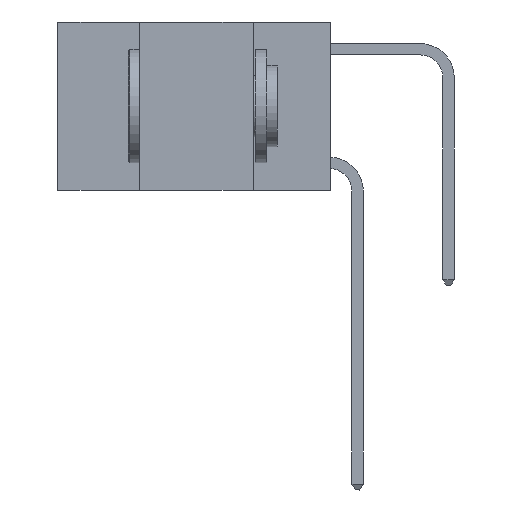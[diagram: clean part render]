
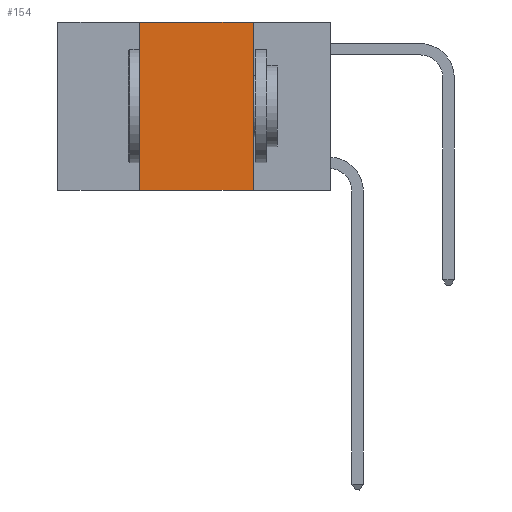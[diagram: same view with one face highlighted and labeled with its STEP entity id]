
A CAD part, left-side view. The second image highlights one B-rep face of the part: STEP entity #154.
In plain terms, the highlighted planar face has unit normal (-1, 0, 0).
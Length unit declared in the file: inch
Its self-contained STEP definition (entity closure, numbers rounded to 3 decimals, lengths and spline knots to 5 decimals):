
#154 = ADVANCED_FACE ( 'NONE', ( #8754 ), #3872, .F. ) ;
#316 = DIRECTION ( 'NONE',  ( 0., -1., 0. ) ) ;
#489 = LINE ( 'NONE', #976, #1999 ) ;
#568 = DIRECTION ( 'NONE',  ( 0., 0., -1. ) ) ;
#976 = CARTESIAN_POINT ( 'NONE',  ( 0., 0.42, 0. ) ) ;
#1014 = DIRECTION ( 'NONE',  ( 0., -1., 0. ) ) ;
#1999 = VECTOR ( 'NONE', #2169, 39.37008 ) ;
#2169 = DIRECTION ( 'NONE',  ( 0., 0., 1. ) ) ;
#2702 = VERTEX_POINT ( 'NONE', #7070 ) ;
#2782 = DIRECTION ( 'NONE',  ( 0., 0., -1. ) ) ;
#3021 = VERTEX_POINT ( 'NONE', #5726 ) ;
#3030 = EDGE_CURVE ( 'NONE', #2702, #3021, #5321, .T. ) ;
#3393 = VECTOR ( 'NONE', #1014, 39.37008 ) ;
#3872 = PLANE ( 'NONE',  #5200 ) ;
#4169 = ORIENTED_EDGE ( 'NONE', *, *, #7814, .T. ) ;
#4462 = VECTOR ( 'NONE', #2782, 39.37008 ) ;
#4655 = VECTOR ( 'NONE', #316, 39.37008 ) ;
#5200 = AXIS2_PLACEMENT_3D ( 'NONE', #6971, #9347, #568 ) ;
#5321 = LINE ( 'NONE', #10060, #4655 ) ;
#5398 = CARTESIAN_POINT ( 'NONE',  ( 0., 0.17, 0. ) ) ;
#5475 = EDGE_LOOP ( 'NONE', ( #6475, #6229, #9011, #4169 ) ) ;
#5726 = CARTESIAN_POINT ( 'NONE',  ( 0., 0.17, 0. ) ) ;
#5914 = VERTEX_POINT ( 'NONE', #9217 ) ;
#6229 = ORIENTED_EDGE ( 'NONE', *, *, #3030, .F. ) ;
#6475 = ORIENTED_EDGE ( 'NONE', *, *, #11972, .F. ) ;
#6971 = CARTESIAN_POINT ( 'NONE',  ( 0., 0.6, 0. ) ) ;
#7070 = CARTESIAN_POINT ( 'NONE',  ( 0., 0.42, 0. ) ) ;
#7090 = LINE ( 'NONE', #7500, #3393 ) ;
#7315 = LINE ( 'NONE', #5398, #4462 ) ;
#7500 = CARTESIAN_POINT ( 'NONE',  ( 0., 0.6, -0.37 ) ) ;
#7814 = EDGE_CURVE ( 'NONE', #5914, #13122, #7090, .T. ) ;
#8754 = FACE_OUTER_BOUND ( 'NONE', #5475, .T. ) ;
#9011 = ORIENTED_EDGE ( 'NONE', *, *, #9287, .F. ) ;
#9217 = CARTESIAN_POINT ( 'NONE',  ( 0., 0.42, -0.37 ) ) ;
#9287 = EDGE_CURVE ( 'NONE', #5914, #2702, #489, .T. ) ;
#9347 = DIRECTION ( 'NONE',  ( 1., 0., 0. ) ) ;
#10060 = CARTESIAN_POINT ( 'NONE',  ( 0., 0.6, 0. ) ) ;
#11972 = EDGE_CURVE ( 'NONE', #3021, #13122, #7315, .T. ) ;
#13122 = VERTEX_POINT ( 'NONE', #13757 ) ;
#13757 = CARTESIAN_POINT ( 'NONE',  ( 0., 0.17, -0.37 ) ) ;
